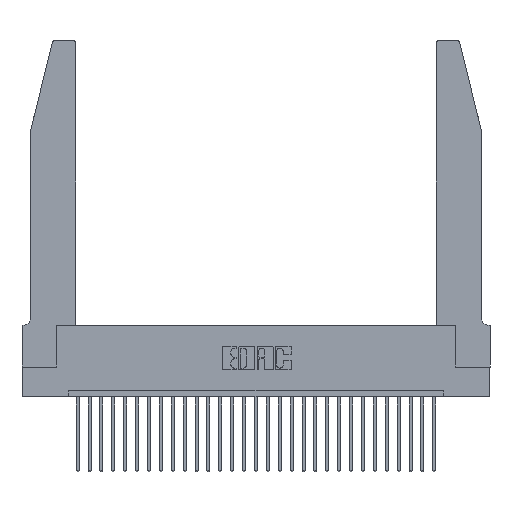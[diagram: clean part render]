
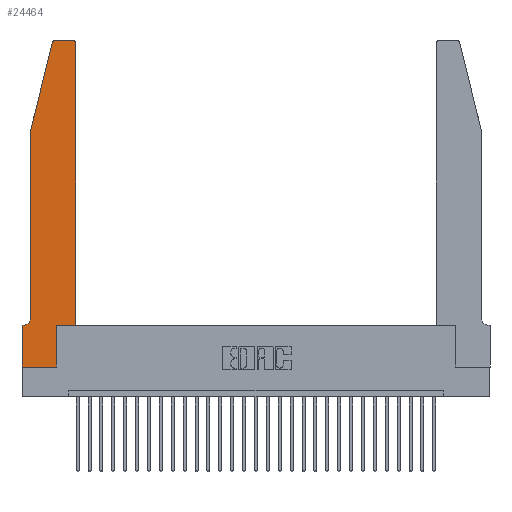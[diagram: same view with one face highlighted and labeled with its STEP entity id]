
A CAD part, top view. The second image highlights one B-rep face of the part: STEP entity #24464.
In plain terms, the highlighted planar face has unit normal (0, 0, 1).
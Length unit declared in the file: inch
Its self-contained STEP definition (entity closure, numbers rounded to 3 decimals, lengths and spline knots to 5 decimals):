
#207 = DIRECTION ( 'NONE',  ( 1., 0., 0. ) ) ;
#495 = EDGE_CURVE ( 'NONE', #9327, #5751, #4074, .T. ) ;
#857 = FACE_OUTER_BOUND ( 'NONE', #19370, .T. ) ;
#901 = CARTESIAN_POINT ( 'NONE',  ( 0.0755, 0.35, 0.37 ) ) ;
#940 = CARTESIAN_POINT ( 'NONE',  ( 0.4505, 0.35, 0.37 ) ) ;
#1271 = EDGE_CURVE ( 'NONE', #29347, #24323, #19423, .T. ) ;
#1614 = LINE ( 'NONE', #940, #10881 ) ;
#1688 = VERTEX_POINT ( 'NONE', #20135 ) ;
#1918 = CARTESIAN_POINT ( 'NONE',  ( 0., 0., 0.37 ) ) ;
#2133 = VERTEX_POINT ( 'NONE', #5154 ) ;
#2339 = ORIENTED_EDGE ( 'NONE', *, *, #25378, .T. ) ;
#2601 = LINE ( 'NONE', #1918, #10098 ) ;
#3605 = EDGE_CURVE ( 'NONE', #1688, #22112, #7140, .T. ) ;
#3797 = VERTEX_POINT ( 'NONE', #13347 ) ;
#4074 = LINE ( 'NONE', #26907, #27329 ) ;
#4739 = CARTESIAN_POINT ( 'NONE',  ( 0.284, 2.72, 0.37 ) ) ;
#5026 = DIRECTION ( 'NONE',  ( 0., 0., 1. ) ) ;
#5154 = CARTESIAN_POINT ( 'NONE',  ( 0.4505, 0.35, 0.37 ) ) ;
#5399 = EDGE_CURVE ( 'NONE', #3797, #18147, #6754, .T. ) ;
#5418 = CARTESIAN_POINT ( 'NONE',  ( 0.0755, 2., 0.37 ) ) ;
#5478 = CIRCLE ( 'NONE', #13252, 0.07 ) ;
#5751 = VERTEX_POINT ( 'NONE', #6586 ) ;
#6004 = DIRECTION ( 'NONE',  ( 1., 0., 0. ) ) ;
#6233 = ORIENTED_EDGE ( 'NONE', *, *, #25055, .T. ) ;
#6308 = VERTEX_POINT ( 'NONE', #11850 ) ;
#6586 = CARTESIAN_POINT ( 'NONE',  ( 0.284, 2.75, 0.37 ) ) ;
#6754 = LINE ( 'NONE', #901, #10685 ) ;
#6983 = CARTESIAN_POINT ( 'NONE',  ( 0.2865, 0.35, 0.37 ) ) ;
#7140 = LINE ( 'NONE', #10936, #14674 ) ;
#8551 = DIRECTION ( 'NONE',  ( 0., 1., 0. ) ) ;
#8996 = DIRECTION ( 'NONE',  ( 0., 1., 0. ) ) ;
#9007 = ORIENTED_EDGE ( 'NONE', *, *, #22853, .T. ) ;
#9055 = ORIENTED_EDGE ( 'NONE', *, *, #3605, .T. ) ;
#9266 = DIRECTION ( 'NONE',  ( 0., -1., 0. ) ) ;
#9327 = VERTEX_POINT ( 'NONE', #23222 ) ;
#9365 = ORIENTED_EDGE ( 'NONE', *, *, #12824, .T. ) ;
#9372 = DIRECTION ( 'NONE',  ( 0., 0., 1. ) ) ;
#9498 = EDGE_CURVE ( 'NONE', #24895, #3797, #5478, .T. ) ;
#9499 = AXIS2_PLACEMENT_3D ( 'NONE', #23054, #9372, #11640 ) ;
#9915 = ORIENTED_EDGE ( 'NONE', *, *, #14412, .T. ) ;
#9979 = CIRCLE ( 'NONE', #20583, 0.03 ) ;
#10098 = VECTOR ( 'NONE', #6004, 39.37008 ) ;
#10232 = DIRECTION ( 'NONE',  ( 0., 0., -1. ) ) ;
#10685 = VECTOR ( 'NONE', #26053, 39.37008 ) ;
#10881 = VECTOR ( 'NONE', #19299, 39.37008 ) ;
#10936 = CARTESIAN_POINT ( 'NONE',  ( 0.0755, 2., 0.37 ) ) ;
#11180 = LINE ( 'NONE', #5418, #29429 ) ;
#11612 = DIRECTION ( 'NONE',  ( 1., 0., 0. ) ) ;
#11640 = DIRECTION ( 'NONE',  ( 1., 0., 0. ) ) ;
#11711 = CARTESIAN_POINT ( 'NONE',  ( 0.0755, 2., 0.37 ) ) ;
#11850 = CARTESIAN_POINT ( 'NONE',  ( 0., 0., 0.37 ) ) ;
#12432 = ORIENTED_EDGE ( 'NONE', *, *, #495, .T. ) ;
#12824 = EDGE_CURVE ( 'NONE', #28871, #9327, #15433, .T. ) ;
#12930 = ORIENTED_EDGE ( 'NONE', *, *, #14302, .T. ) ;
#13252 = AXIS2_PLACEMENT_3D ( 'NONE', #17048, #10232, #26807 ) ;
#13347 = CARTESIAN_POINT ( 'NONE',  ( 0.0055, 0.35, 0.37 ) ) ;
#13496 = CARTESIAN_POINT ( 'NONE',  ( 0., 0.35, 0.37 ) ) ;
#13672 = DIRECTION ( 'NONE',  ( 0., 0., 1. ) ) ;
#14302 = EDGE_CURVE ( 'NONE', #5751, #1688, #9979, .T. ) ;
#14412 = EDGE_CURVE ( 'NONE', #2133, #28871, #14984, .T. ) ;
#14614 = DIRECTION ( 'NONE',  ( 0., -1., 0. ) ) ;
#14674 = VECTOR ( 'NONE', #21446, 39.37008 ) ;
#14926 = CARTESIAN_POINT ( 'NONE',  ( 0.4505, 0.35, 0.37 ) ) ;
#14984 = LINE ( 'NONE', #14926, #20310 ) ;
#15433 = CIRCLE ( 'NONE', #22312, 0.03 ) ;
#16934 = ORIENTED_EDGE ( 'NONE', *, *, #5399, .T. ) ;
#17048 = CARTESIAN_POINT ( 'NONE',  ( 0.0055, 0.42, 0.37 ) ) ;
#17650 = CARTESIAN_POINT ( 'NONE',  ( 0.2865, 0., 0.37 ) ) ;
#18147 = VERTEX_POINT ( 'NONE', #13496 ) ;
#19298 = CARTESIAN_POINT ( 'NONE',  ( 0.4505, 2.72, 0.37 ) ) ;
#19299 = DIRECTION ( 'NONE',  ( 1., 0., 0. ) ) ;
#19370 = EDGE_LOOP ( 'NONE', ( #12432, #12930, #9055, #6233, #28486, #16934, #9007, #2339, #28076, #19884, #9915, #9365 ) ) ;
#19423 = LINE ( 'NONE', #6983, #20452 ) ;
#19884 = ORIENTED_EDGE ( 'NONE', *, *, #24130, .T. ) ;
#20135 = CARTESIAN_POINT ( 'NONE',  ( 0.25487, 2.72718, 0.37 ) ) ;
#20234 = CARTESIAN_POINT ( 'NONE',  ( 0.2865, 0.35, 0.37 ) ) ;
#20310 = VECTOR ( 'NONE', #8551, 39.37008 ) ;
#20452 = VECTOR ( 'NONE', #8996, 39.37008 ) ;
#20583 = AXIS2_PLACEMENT_3D ( 'NONE', #4739, #5026, #11612 ) ;
#20719 = CARTESIAN_POINT ( 'NONE',  ( 0., 0., 0.37 ) ) ;
#21446 = DIRECTION ( 'NONE',  ( -0.239, -0.971, 0. ) ) ;
#21631 = LINE ( 'NONE', #20719, #23068 ) ;
#22112 = VERTEX_POINT ( 'NONE', #11711 ) ;
#22312 = AXIS2_PLACEMENT_3D ( 'NONE', #23063, #13672, #207 ) ;
#22757 = PLANE ( 'NONE',  #9499 ) ;
#22853 = EDGE_CURVE ( 'NONE', #18147, #6308, #21631, .T. ) ;
#23054 = CARTESIAN_POINT ( 'NONE',  ( 0., 0.35, 0.37 ) ) ;
#23063 = CARTESIAN_POINT ( 'NONE',  ( 0.4205, 2.72, 0.37 ) ) ;
#23068 = VECTOR ( 'NONE', #9266, 39.37008 ) ;
#23222 = CARTESIAN_POINT ( 'NONE',  ( 0.4205, 2.75, 0.37 ) ) ;
#24130 = EDGE_CURVE ( 'NONE', #24323, #2133, #1614, .T. ) ;
#24323 = VERTEX_POINT ( 'NONE', #20234 ) ;
#24464 = ADVANCED_FACE ( 'NONE', ( #857 ), #22757, .T. ) ;
#24607 = DIRECTION ( 'NONE',  ( -1., 0., 0. ) ) ;
#24895 = VERTEX_POINT ( 'NONE', #27106 ) ;
#25055 = EDGE_CURVE ( 'NONE', #22112, #24895, #11180, .T. ) ;
#25378 = EDGE_CURVE ( 'NONE', #6308, #29347, #2601, .T. ) ;
#26053 = DIRECTION ( 'NONE',  ( -1., 0., 0. ) ) ;
#26807 = DIRECTION ( 'NONE',  ( -1., 0., 0. ) ) ;
#26907 = CARTESIAN_POINT ( 'NONE',  ( 0.2605, 2.75, 0.37 ) ) ;
#27106 = CARTESIAN_POINT ( 'NONE',  ( 0.0755, 0.42, 0.37 ) ) ;
#27329 = VECTOR ( 'NONE', #24607, 39.37008 ) ;
#28076 = ORIENTED_EDGE ( 'NONE', *, *, #1271, .T. ) ;
#28486 = ORIENTED_EDGE ( 'NONE', *, *, #9498, .T. ) ;
#28871 = VERTEX_POINT ( 'NONE', #19298 ) ;
#29347 = VERTEX_POINT ( 'NONE', #17650 ) ;
#29429 = VECTOR ( 'NONE', #14614, 39.37008 ) ;
